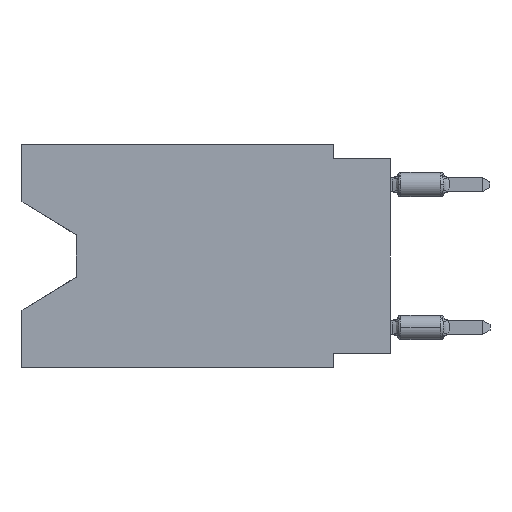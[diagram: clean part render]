
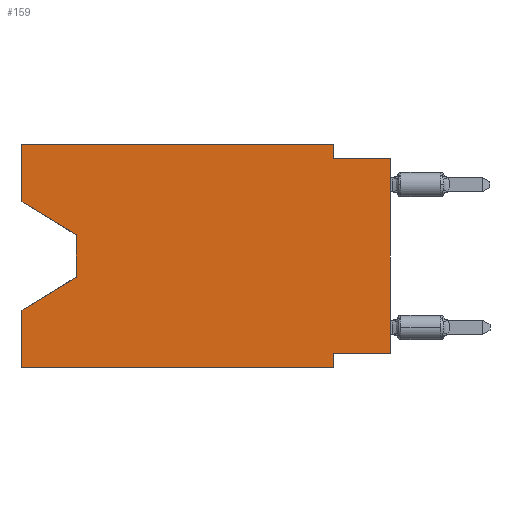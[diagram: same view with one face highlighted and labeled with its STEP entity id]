
A CAD part, left-side view. The second image highlights one B-rep face of the part: STEP entity #159.
In plain terms, the highlighted planar face has unit normal (-1, 0, 0).
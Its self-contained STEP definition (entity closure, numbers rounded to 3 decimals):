
#159 = ADVANCED_FACE ( 'NONE', ( #9645 ), #12805, .F. ) ;
#352 = DIRECTION ( 'NONE',  ( 0., 0.855, -0.519 ) ) ;
#442 = CARTESIAN_POINT ( 'NONE',  ( 0., 0., -0.635 ) ) ;
#675 = CARTESIAN_POINT ( 'NONE',  ( 0., 13.97, -5.893 ) ) ;
#702 = CARTESIAN_POINT ( 'NONE',  ( 0., 16.383, -2.546 ) ) ;
#713 = LINE ( 'NONE', #10116, #13186 ) ;
#1110 = DIRECTION ( 'NONE',  ( 0., 0., 1. ) ) ;
#1307 = CARTESIAN_POINT ( 'NONE',  ( 0., 0., -9.271 ) ) ;
#1677 = ORIENTED_EDGE ( 'NONE', *, *, #8840, .F. ) ;
#1765 = AXIS2_PLACEMENT_3D ( 'NONE', #1884, #8127, #3643 ) ;
#1884 = CARTESIAN_POINT ( 'NONE',  ( 0., 16.383, 0. ) ) ;
#2190 = VERTEX_POINT ( 'NONE', #6803 ) ;
#2346 = ORIENTED_EDGE ( 'NONE', *, *, #9816, .F. ) ;
#2387 = ORIENTED_EDGE ( 'NONE', *, *, #15813, .T. ) ;
#2467 = CARTESIAN_POINT ( 'NONE',  ( 0., 16.383, -2.546 ) ) ;
#2594 = ORIENTED_EDGE ( 'NONE', *, *, #6931, .F. ) ;
#2596 = CARTESIAN_POINT ( 'NONE',  ( 0., 16.383, -9.906 ) ) ;
#2659 = CARTESIAN_POINT ( 'NONE',  ( 0., 13.97, -4.013 ) ) ;
#2712 = EDGE_CURVE ( 'NONE', #4837, #9263, #13590, .T. ) ;
#2932 = VECTOR ( 'NONE', #9549, 1000. ) ;
#3643 = DIRECTION ( 'NONE',  ( 0., 0., -1. ) ) ;
#3970 = VERTEX_POINT ( 'NONE', #2467 ) ;
#4195 = CARTESIAN_POINT ( 'NONE',  ( 0., 2.54, -9.271 ) ) ;
#4251 = CARTESIAN_POINT ( 'NONE',  ( 0., 2.54, -9.906 ) ) ;
#4305 = LINE ( 'NONE', #15702, #7084 ) ;
#4445 = LINE ( 'NONE', #16850, #8150 ) ;
#4526 = EDGE_CURVE ( 'NONE', #3970, #8431, #20165, .T. ) ;
#4584 = ORIENTED_EDGE ( 'NONE', *, *, #8035, .F. ) ;
#4837 = VERTEX_POINT ( 'NONE', #14037 ) ;
#4909 = LINE ( 'NONE', #18938, #7970 ) ;
#4929 = DIRECTION ( 'NONE',  ( 0., -0.855, -0.519 ) ) ;
#5006 = DIRECTION ( 'NONE',  ( 0., 0., -1. ) ) ;
#5394 = VECTOR ( 'NONE', #19116, 1000. ) ;
#5955 = CARTESIAN_POINT ( 'NONE',  ( 0., 16.383, 0. ) ) ;
#6089 = EDGE_CURVE ( 'NONE', #3970, #16669, #13070, .T. ) ;
#6161 = ORIENTED_EDGE ( 'NONE', *, *, #9915, .T. ) ;
#6228 = VERTEX_POINT ( 'NONE', #4195 ) ;
#6347 = VECTOR ( 'NONE', #1110, 1000. ) ;
#6541 = EDGE_CURVE ( 'NONE', #6228, #14930, #4909, .T. ) ;
#6803 = CARTESIAN_POINT ( 'NONE',  ( 0., 0., -0.635 ) ) ;
#6931 = EDGE_CURVE ( 'NONE', #19212, #2190, #17584, .T. ) ;
#6973 = DIRECTION ( 'NONE',  ( 0., 0., 1. ) ) ;
#7084 = VECTOR ( 'NONE', #15517, 1000. ) ;
#7557 = CARTESIAN_POINT ( 'NONE',  ( 0., 16.383, -7.36 ) ) ;
#7963 = ORIENTED_EDGE ( 'NONE', *, *, #13844, .T. ) ;
#7970 = VECTOR ( 'NONE', #5006, 1000. ) ;
#8016 = ORIENTED_EDGE ( 'NONE', *, *, #2712, .F. ) ;
#8035 = EDGE_CURVE ( 'NONE', #14208, #6228, #14356, .T. ) ;
#8127 = DIRECTION ( 'NONE',  ( 1., 0., 0. ) ) ;
#8150 = VECTOR ( 'NONE', #10751, 1000. ) ;
#8431 = VERTEX_POINT ( 'NONE', #18984 ) ;
#8745 = ORIENTED_EDGE ( 'NONE', *, *, #6541, .F. ) ;
#8840 = EDGE_CURVE ( 'NONE', #10155, #19212, #4305, .T. ) ;
#8849 = EDGE_LOOP ( 'NONE', ( #11331, #7963, #17246, #8016, #6161, #8745, #4584, #2387, #2594, #1677, #2346, #15421 ) ) ;
#9263 = VERTEX_POINT ( 'NONE', #7557 ) ;
#9319 = VERTEX_POINT ( 'NONE', #675 ) ;
#9549 = DIRECTION ( 'NONE',  ( 0., 0., 1. ) ) ;
#9634 = VECTOR ( 'NONE', #18911, 1000. ) ;
#9645 = FACE_OUTER_BOUND ( 'NONE', #8849, .T. ) ;
#9679 = VECTOR ( 'NONE', #16163, 1000. ) ;
#9816 = EDGE_CURVE ( 'NONE', #8431, #10155, #11174, .T. ) ;
#9850 = CARTESIAN_POINT ( 'NONE',  ( 0., 0., -9.271 ) ) ;
#9915 = EDGE_CURVE ( 'NONE', #4837, #14930, #10152, .T. ) ;
#10116 = CARTESIAN_POINT ( 'NONE',  ( 0., 0., 0. ) ) ;
#10152 = LINE ( 'NONE', #2596, #17821 ) ;
#10155 = VERTEX_POINT ( 'NONE', #15909 ) ;
#10546 = VECTOR ( 'NONE', #4929, 1000. ) ;
#10751 = DIRECTION ( 'NONE',  ( 0., 0., -1. ) ) ;
#11174 = LINE ( 'NONE', #17685, #9679 ) ;
#11331 = ORIENTED_EDGE ( 'NONE', *, *, #6089, .T. ) ;
#12180 = EDGE_CURVE ( 'NONE', #9319, #9263, #12926, .T. ) ;
#12805 = PLANE ( 'NONE',  #1765 ) ;
#12926 = LINE ( 'NONE', #14678, #13411 ) ;
#13070 = LINE ( 'NONE', #702, #10546 ) ;
#13186 = VECTOR ( 'NONE', #6973, 1000. ) ;
#13411 = VECTOR ( 'NONE', #352, 1000. ) ;
#13590 = LINE ( 'NONE', #5955, #6347 ) ;
#13844 = EDGE_CURVE ( 'NONE', #16669, #9319, #4445, .T. ) ;
#14037 = CARTESIAN_POINT ( 'NONE',  ( 0., 16.383, -9.906 ) ) ;
#14208 = VERTEX_POINT ( 'NONE', #1307 ) ;
#14313 = CARTESIAN_POINT ( 'NONE',  ( 0., 2.54, -0.635 ) ) ;
#14356 = LINE ( 'NONE', #9850, #9634 ) ;
#14678 = CARTESIAN_POINT ( 'NONE',  ( 0., 13.97, -5.893 ) ) ;
#14762 = DIRECTION ( 'NONE',  ( 0., -1., 0. ) ) ;
#14930 = VERTEX_POINT ( 'NONE', #4251 ) ;
#15421 = ORIENTED_EDGE ( 'NONE', *, *, #4526, .F. ) ;
#15517 = DIRECTION ( 'NONE',  ( 0., 0., -1. ) ) ;
#15702 = CARTESIAN_POINT ( 'NONE',  ( 0., 2.54, 0. ) ) ;
#15813 = EDGE_CURVE ( 'NONE', #14208, #2190, #713, .T. ) ;
#15909 = CARTESIAN_POINT ( 'NONE',  ( 0., 2.54, 0. ) ) ;
#16163 = DIRECTION ( 'NONE',  ( 0., -1., 0. ) ) ;
#16669 = VERTEX_POINT ( 'NONE', #2659 ) ;
#16850 = CARTESIAN_POINT ( 'NONE',  ( 0., 13.97, -4.013 ) ) ;
#17246 = ORIENTED_EDGE ( 'NONE', *, *, #12180, .T. ) ;
#17584 = LINE ( 'NONE', #442, #5394 ) ;
#17685 = CARTESIAN_POINT ( 'NONE',  ( 0., 16.383, 0. ) ) ;
#17821 = VECTOR ( 'NONE', #14762, 1000. ) ;
#18412 = CARTESIAN_POINT ( 'NONE',  ( 0., 16.383, 0. ) ) ;
#18911 = DIRECTION ( 'NONE',  ( 0., 1., 0. ) ) ;
#18938 = CARTESIAN_POINT ( 'NONE',  ( 0., 2.54, -9.906 ) ) ;
#18984 = CARTESIAN_POINT ( 'NONE',  ( 0., 16.383, 0. ) ) ;
#19116 = DIRECTION ( 'NONE',  ( 0., -1., 0. ) ) ;
#19212 = VERTEX_POINT ( 'NONE', #14313 ) ;
#20165 = LINE ( 'NONE', #18412, #2932 ) ;
